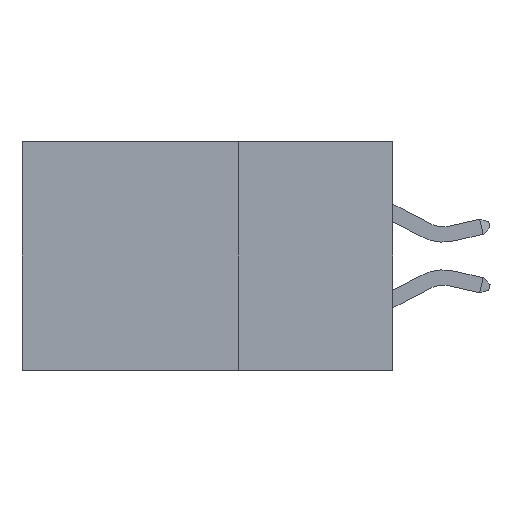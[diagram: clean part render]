
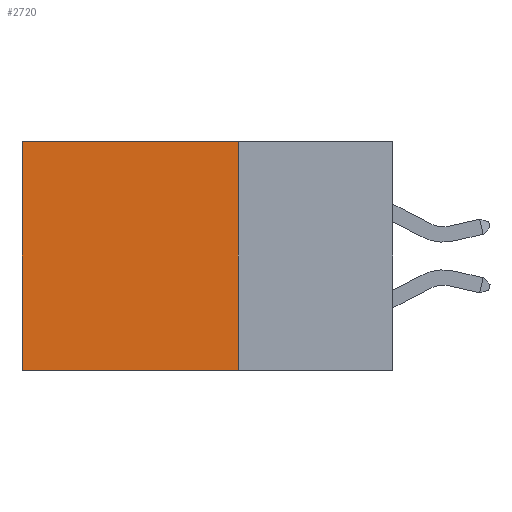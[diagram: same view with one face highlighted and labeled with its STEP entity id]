
A CAD part, left-side view. The second image highlights one B-rep face of the part: STEP entity #2720.
In plain terms, the highlighted planar face has unit normal (-1, 0, 0).
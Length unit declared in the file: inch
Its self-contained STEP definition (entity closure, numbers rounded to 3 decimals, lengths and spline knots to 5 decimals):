
#111 = EDGE_CURVE ( 'NONE', #9295, #16756, #3762, .T. ) ;
#620 = CARTESIAN_POINT ( 'NONE',  ( 0.2875, 0.25, -0.37 ) ) ;
#1002 = DIRECTION ( 'NONE',  ( 0., 0., -1. ) ) ;
#1535 = LINE ( 'NONE', #620, #6636 ) ;
#1987 = DIRECTION ( 'NONE',  ( 0., 1., 0. ) ) ;
#2213 = LINE ( 'NONE', #15335, #15522 ) ;
#2720 = ADVANCED_FACE ( 'NONE', ( #9997 ), #5550, .F. ) ;
#3073 = EDGE_CURVE ( 'NONE', #16756, #9307, #1535, .T. ) ;
#3762 = LINE ( 'NONE', #5465, #15129 ) ;
#4202 = CARTESIAN_POINT ( 'NONE',  ( 0.2875, 0.25, 0. ) ) ;
#5465 = CARTESIAN_POINT ( 'NONE',  ( 0.2875, 0.25, 0. ) ) ;
#5550 = PLANE ( 'NONE',  #12732 ) ;
#5706 = ORIENTED_EDGE ( 'NONE', *, *, #13875, .T. ) ;
#6636 = VECTOR ( 'NONE', #1987, 39.37008 ) ;
#6914 = DIRECTION ( 'NONE',  ( 1., 0., 0. ) ) ;
#7061 = CARTESIAN_POINT ( 'NONE',  ( 0.2875, 0.6, 0. ) ) ;
#7099 = LINE ( 'NONE', #17055, #11107 ) ;
#7427 = VERTEX_POINT ( 'NONE', #7061 ) ;
#8143 = CARTESIAN_POINT ( 'NONE',  ( 0.2875, 0.6, -0.37 ) ) ;
#8314 = DIRECTION ( 'NONE',  ( 0., 0., -1. ) ) ;
#8837 = ORIENTED_EDGE ( 'NONE', *, *, #13942, .T. ) ;
#9295 = VERTEX_POINT ( 'NONE', #16034 ) ;
#9307 = VERTEX_POINT ( 'NONE', #8143 ) ;
#9926 = DIRECTION ( 'NONE',  ( 0., 0., -1. ) ) ;
#9997 = FACE_OUTER_BOUND ( 'NONE', #12546, .T. ) ;
#10622 = ORIENTED_EDGE ( 'NONE', *, *, #3073, .F. ) ;
#11107 = VECTOR ( 'NONE', #1002, 39.37008 ) ;
#12414 = ORIENTED_EDGE ( 'NONE', *, *, #111, .F. ) ;
#12546 = EDGE_LOOP ( 'NONE', ( #8837, #10622, #12414, #5706 ) ) ;
#12727 = DIRECTION ( 'NONE',  ( 0., 1., 0. ) ) ;
#12732 = AXIS2_PLACEMENT_3D ( 'NONE', #4202, #6914, #8314 ) ;
#13875 = EDGE_CURVE ( 'NONE', #9295, #7427, #2213, .T. ) ;
#13942 = EDGE_CURVE ( 'NONE', #7427, #9307, #7099, .T. ) ;
#15129 = VECTOR ( 'NONE', #9926, 39.37008 ) ;
#15335 = CARTESIAN_POINT ( 'NONE',  ( 0.2875, 0.25, 0. ) ) ;
#15522 = VECTOR ( 'NONE', #12727, 39.37008 ) ;
#16034 = CARTESIAN_POINT ( 'NONE',  ( 0.2875, 0.25, 0. ) ) ;
#16649 = CARTESIAN_POINT ( 'NONE',  ( 0.2875, 0.25, -0.37 ) ) ;
#16756 = VERTEX_POINT ( 'NONE', #16649 ) ;
#17055 = CARTESIAN_POINT ( 'NONE',  ( 0.2875, 0.6, 0. ) ) ;
